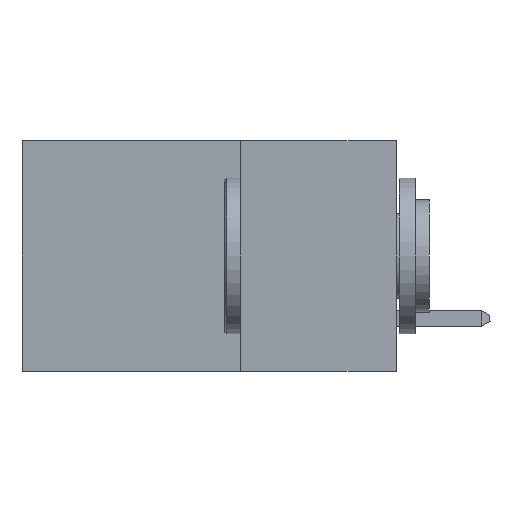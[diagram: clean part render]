
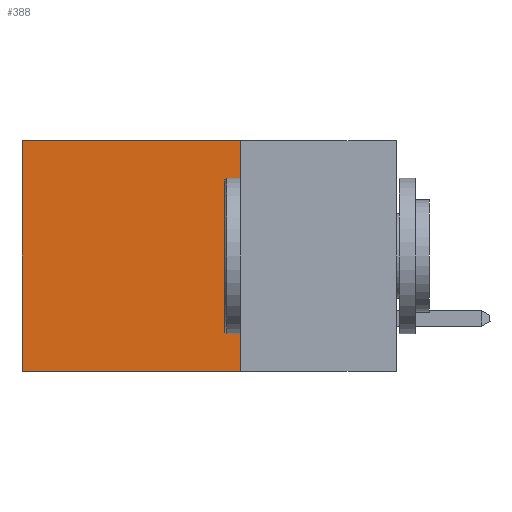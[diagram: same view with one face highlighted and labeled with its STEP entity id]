
A CAD part, left-side view. The second image highlights one B-rep face of the part: STEP entity #388.
In plain terms, the highlighted planar face has unit normal (-1, 0, 0).
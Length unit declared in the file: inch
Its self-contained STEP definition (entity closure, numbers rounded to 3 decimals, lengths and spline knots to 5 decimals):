
#225 = LINE ( 'NONE', #3982, #4443 ) ;
#339 = DIRECTION ( 'NONE',  ( 0., 0., -1. ) ) ;
#388 = ADVANCED_FACE ( 'NONE', ( #3133 ), #10386, .F. ) ;
#433 = VERTEX_POINT ( 'NONE', #7683 ) ;
#596 = DIRECTION ( 'NONE',  ( 1., 0., 0. ) ) ;
#1111 = CARTESIAN_POINT ( 'NONE',  ( 0.298, 0.6, 0. ) ) ;
#1404 = EDGE_CURVE ( 'NONE', #433, #7213, #225, .T. ) ;
#1609 = LINE ( 'NONE', #4868, #9900 ) ;
#1711 = EDGE_LOOP ( 'NONE', ( #4119, #9598, #2312, #7760 ) ) ;
#2312 = ORIENTED_EDGE ( 'NONE', *, *, #1404, .F. ) ;
#2747 = EDGE_CURVE ( 'NONE', #433, #9883, #1609, .T. ) ;
#3133 = FACE_OUTER_BOUND ( 'NONE', #1711, .T. ) ;
#3201 = DIRECTION ( 'NONE',  ( 0., 1., 0. ) ) ;
#3562 = AXIS2_PLACEMENT_3D ( 'NONE', #4944, #596, #8516 ) ;
#3609 = CARTESIAN_POINT ( 'NONE',  ( 0.298, 0.25, -0.37 ) ) ;
#3664 = EDGE_CURVE ( 'NONE', #7213, #4028, #9275, .T. ) ;
#3982 = CARTESIAN_POINT ( 'NONE',  ( 0.298, 0.25, 0. ) ) ;
#4007 = LINE ( 'NONE', #1111, #10243 ) ;
#4028 = VERTEX_POINT ( 'NONE', #9771 ) ;
#4119 = ORIENTED_EDGE ( 'NONE', *, *, #4909, .T. ) ;
#4443 = VECTOR ( 'NONE', #4454, 39.37008 ) ;
#4454 = DIRECTION ( 'NONE',  ( 0., 0., -1. ) ) ;
#4868 = CARTESIAN_POINT ( 'NONE',  ( 0.298, 0.25, 0. ) ) ;
#4909 = EDGE_CURVE ( 'NONE', #9883, #4028, #4007, .T. ) ;
#4944 = CARTESIAN_POINT ( 'NONE',  ( 0.298, 0.25, 0. ) ) ;
#5068 = DIRECTION ( 'NONE',  ( 0., 1., 0. ) ) ;
#5700 = CARTESIAN_POINT ( 'NONE',  ( 0.298, 0.6, 0. ) ) ;
#7114 = VECTOR ( 'NONE', #3201, 39.37008 ) ;
#7213 = VERTEX_POINT ( 'NONE', #8957 ) ;
#7683 = CARTESIAN_POINT ( 'NONE',  ( 0.298, 0.25, 0. ) ) ;
#7760 = ORIENTED_EDGE ( 'NONE', *, *, #2747, .T. ) ;
#8516 = DIRECTION ( 'NONE',  ( 0., 0., -1. ) ) ;
#8957 = CARTESIAN_POINT ( 'NONE',  ( 0.298, 0.25, -0.37 ) ) ;
#9275 = LINE ( 'NONE', #3609, #7114 ) ;
#9598 = ORIENTED_EDGE ( 'NONE', *, *, #3664, .F. ) ;
#9771 = CARTESIAN_POINT ( 'NONE',  ( 0.298, 0.6, -0.37 ) ) ;
#9883 = VERTEX_POINT ( 'NONE', #5700 ) ;
#9900 = VECTOR ( 'NONE', #5068, 39.37008 ) ;
#10243 = VECTOR ( 'NONE', #339, 39.37008 ) ;
#10386 = PLANE ( 'NONE',  #3562 ) ;
